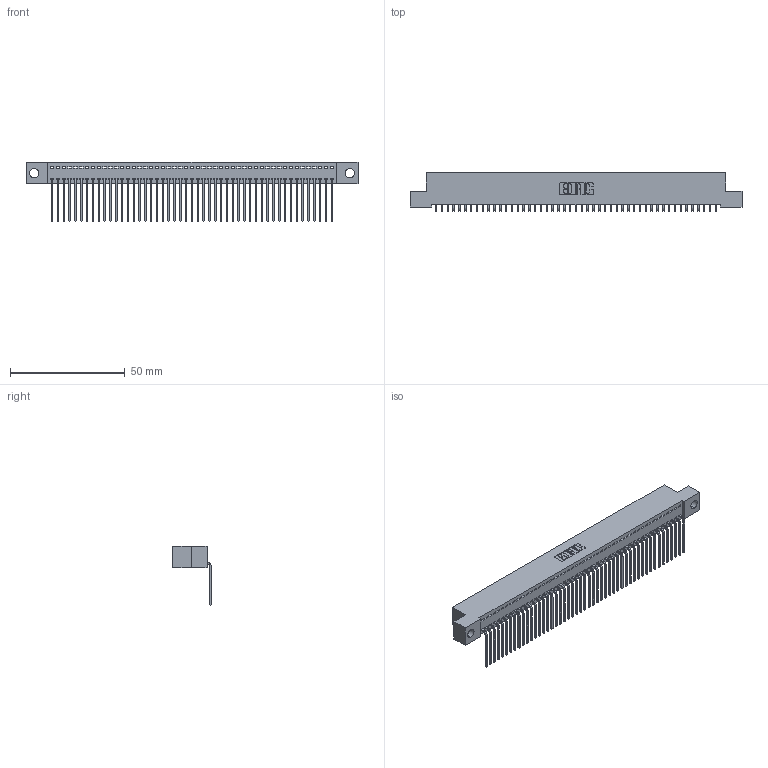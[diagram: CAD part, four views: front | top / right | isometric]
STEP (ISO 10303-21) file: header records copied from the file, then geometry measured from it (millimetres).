
FILE_DESCRIPTION (( 'STEP AP203' ), '1' );
FILE_NAME ('392-049-559-104.STEP', '2019-10-08T11:00:55', ( '' ), ( '' ), 'SwSTEP 2.0', 'SolidWorks 2016', '' );
FILE_SCHEMA (( 'CONFIG_CONTROL_DESIGN' ));
Length unit declared in the file: inch
Products named in the file (3): 342 Part_.156 TH; 345-292-001_558 559 Tail - 1; 392-049-559-104
Assembly tree (50 placements, depth 2):
  392-049-559-104
    342 Part_.156 TH
    345-292-001_558 559 Tail - 1  x49
Bounding box: 144.78 x 16.83 x 25.78 mm (x, y, z)
Volume: 12796.3 mm3; surface area: 19667.5 mm2
Topology: 50 solids, 50 shells, 3050 faces, 9217 edges, 6078 vertices
Faces by surface type: plane 2222, cylinder 828
Entity records: 29005 total; most frequent: CARTESIAN_POINT 5009, ORIENTED_EDGE 4994, DIRECTION 4211, EDGE_CURVE 2497, VECTOR 2369, LINE 2369, VERTEX_POINT 1662, AXIS2_PLACEMENT_3D 921
